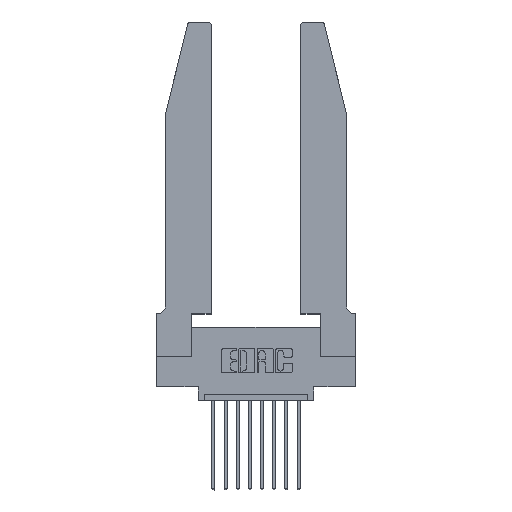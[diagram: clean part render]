
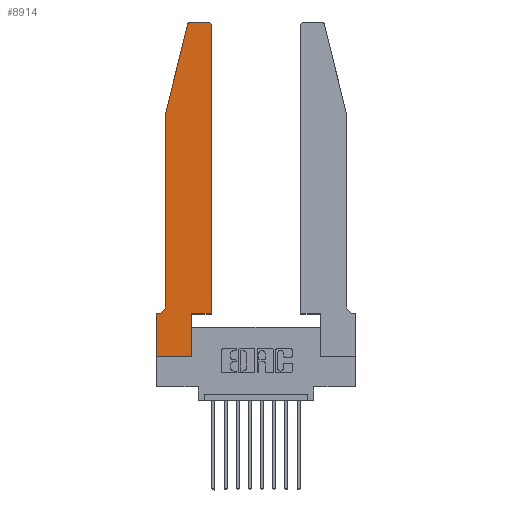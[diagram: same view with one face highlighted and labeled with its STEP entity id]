
A CAD part, top view. The second image highlights one B-rep face of the part: STEP entity #8914.
In plain terms, the highlighted planar face has unit normal (0, 0, 1).
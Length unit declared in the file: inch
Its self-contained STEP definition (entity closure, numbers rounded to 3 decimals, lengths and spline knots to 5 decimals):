
#703 = DIRECTION ( 'NONE',  ( 1., 0., 0. ) ) ;
#865 = VECTOR ( 'NONE', #4171, 39.37008 ) ;
#1129 = CARTESIAN_POINT ( 'NONE',  ( 0.284, 2.72, 0.37 ) ) ;
#1334 = ORIENTED_EDGE ( 'NONE', *, *, #7457, .T. ) ;
#1500 = ORIENTED_EDGE ( 'NONE', *, *, #13188, .T. ) ;
#1532 = CARTESIAN_POINT ( 'NONE',  ( 0.0755, 0.42, 0.37 ) ) ;
#1730 = CIRCLE ( 'NONE', #3489, 0.03 ) ;
#1810 = CARTESIAN_POINT ( 'NONE',  ( 0., 0., 0.37 ) ) ;
#2021 = DIRECTION ( 'NONE',  ( 0., 0., 1. ) ) ;
#2059 = LINE ( 'NONE', #1810, #7297 ) ;
#2123 = ORIENTED_EDGE ( 'NONE', *, *, #7817, .T. ) ;
#2162 = CARTESIAN_POINT ( 'NONE',  ( 0.2865, 0.35, 0.37 ) ) ;
#2186 = DIRECTION ( 'NONE',  ( -1., 0., 0. ) ) ;
#2291 = EDGE_LOOP ( 'NONE', ( #1500, #11821, #11492, #4103, #11208, #12050, #1334, #4428, #11023, #2123, #2442, #6699 ) ) ;
#2324 = CARTESIAN_POINT ( 'NONE',  ( 0.4205, 2.75, 0.37 ) ) ;
#2404 = DIRECTION ( 'NONE',  ( 0., 1., 0. ) ) ;
#2442 = ORIENTED_EDGE ( 'NONE', *, *, #6594, .T. ) ;
#2480 = CARTESIAN_POINT ( 'NONE',  ( 0.0755, 2., 0.37 ) ) ;
#2630 = CARTESIAN_POINT ( 'NONE',  ( 0., 0., 0.37 ) ) ;
#2675 = CARTESIAN_POINT ( 'NONE',  ( 0., 0., 0.37 ) ) ;
#2876 = VECTOR ( 'NONE', #4924, 39.37008 ) ;
#3134 = VECTOR ( 'NONE', #4194, 39.37008 ) ;
#3347 = VERTEX_POINT ( 'NONE', #7876 ) ;
#3489 = AXIS2_PLACEMENT_3D ( 'NONE', #6649, #2021, #703 ) ;
#3671 = FACE_OUTER_BOUND ( 'NONE', #2291, .T. ) ;
#4103 = ORIENTED_EDGE ( 'NONE', *, *, #8977, .T. ) ;
#4171 = DIRECTION ( 'NONE',  ( 0., -1., 0. ) ) ;
#4194 = DIRECTION ( 'NONE',  ( 0., 1., 0. ) ) ;
#4280 = EDGE_CURVE ( 'NONE', #15359, #8386, #5883, .T. ) ;
#4428 = ORIENTED_EDGE ( 'NONE', *, *, #14507, .T. ) ;
#4581 = AXIS2_PLACEMENT_3D ( 'NONE', #5215, #9995, #13709 ) ;
#4614 = VERTEX_POINT ( 'NONE', #8157 ) ;
#4744 = DIRECTION ( 'NONE',  ( -1., 0., 0. ) ) ;
#4924 = DIRECTION ( 'NONE',  ( -0.239, -0.971, 0. ) ) ;
#4974 = CARTESIAN_POINT ( 'NONE',  ( 0.4505, 0.35, 0.37 ) ) ;
#5093 = VECTOR ( 'NONE', #2404, 39.37008 ) ;
#5166 = CARTESIAN_POINT ( 'NONE',  ( 0.0055, 0.35, 0.37 ) ) ;
#5215 = CARTESIAN_POINT ( 'NONE',  ( 0.0055, 0.42, 0.37 ) ) ;
#5605 = CARTESIAN_POINT ( 'NONE',  ( 0., 0.35, 0.37 ) ) ;
#5632 = EDGE_CURVE ( 'NONE', #3347, #9350, #1730, .T. ) ;
#5797 = EDGE_CURVE ( 'NONE', #4614, #12035, #6051, .T. ) ;
#5883 = CIRCLE ( 'NONE', #4581, 0.07 ) ;
#5971 = DIRECTION ( 'NONE',  ( 1., 0., 0. ) ) ;
#5994 = LINE ( 'NONE', #2675, #7677 ) ;
#6051 = LINE ( 'NONE', #7262, #2876 ) ;
#6124 = DIRECTION ( 'NONE',  ( 0., 0., 1. ) ) ;
#6227 = VERTEX_POINT ( 'NONE', #13245 ) ;
#6325 = LINE ( 'NONE', #6650, #3134 ) ;
#6479 = CARTESIAN_POINT ( 'NONE',  ( 0., 0.35, 0.37 ) ) ;
#6594 = EDGE_CURVE ( 'NONE', #14875, #3347, #8634, .T. ) ;
#6649 = CARTESIAN_POINT ( 'NONE',  ( 0.4205, 2.72, 0.37 ) ) ;
#6650 = CARTESIAN_POINT ( 'NONE',  ( 0.2865, 0.35, 0.37 ) ) ;
#6699 = ORIENTED_EDGE ( 'NONE', *, *, #5632, .T. ) ;
#6800 = DIRECTION ( 'NONE',  ( 1., 0., 0. ) ) ;
#6939 = LINE ( 'NONE', #9329, #9908 ) ;
#7262 = CARTESIAN_POINT ( 'NONE',  ( 0.0755, 2., 0.37 ) ) ;
#7297 = VECTOR ( 'NONE', #8869, 39.37008 ) ;
#7308 = VECTOR ( 'NONE', #4744, 39.37008 ) ;
#7457 = EDGE_CURVE ( 'NONE', #13392, #14894, #5994, .T. ) ;
#7660 = VECTOR ( 'NONE', #5971, 39.37008 ) ;
#7677 = VECTOR ( 'NONE', #12021, 39.37008 ) ;
#7817 = EDGE_CURVE ( 'NONE', #14846, #14875, #9886, .T. ) ;
#7876 = CARTESIAN_POINT ( 'NONE',  ( 0.4505, 2.72, 0.37 ) ) ;
#8157 = CARTESIAN_POINT ( 'NONE',  ( 0.25487, 2.72718, 0.37 ) ) ;
#8386 = VERTEX_POINT ( 'NONE', #5166 ) ;
#8634 = LINE ( 'NONE', #4974, #5093 ) ;
#8869 = DIRECTION ( 'NONE',  ( 1., 0., 0. ) ) ;
#8914 = ADVANCED_FACE ( 'NONE', ( #3671 ), #11519, .T. ) ;
#8977 = EDGE_CURVE ( 'NONE', #12035, #15359, #13587, .T. ) ;
#9088 = EDGE_CURVE ( 'NONE', #9193, #14846, #6325, .T. ) ;
#9178 = CARTESIAN_POINT ( 'NONE',  ( 0.0755, 2., 0.37 ) ) ;
#9193 = VERTEX_POINT ( 'NONE', #14758 ) ;
#9329 = CARTESIAN_POINT ( 'NONE',  ( 0.2605, 2.75, 0.37 ) ) ;
#9350 = VERTEX_POINT ( 'NONE', #2324 ) ;
#9886 = LINE ( 'NONE', #13187, #7660 ) ;
#9908 = VECTOR ( 'NONE', #2186, 39.37008 ) ;
#9995 = DIRECTION ( 'NONE',  ( 0., 0., -1. ) ) ;
#10645 = LINE ( 'NONE', #12028, #7308 ) ;
#10739 = DIRECTION ( 'NONE',  ( 1., 0., 0. ) ) ;
#11023 = ORIENTED_EDGE ( 'NONE', *, *, #9088, .T. ) ;
#11053 = AXIS2_PLACEMENT_3D ( 'NONE', #5605, #13994, #6800 ) ;
#11208 = ORIENTED_EDGE ( 'NONE', *, *, #4280, .T. ) ;
#11492 = ORIENTED_EDGE ( 'NONE', *, *, #5797, .T. ) ;
#11519 = PLANE ( 'NONE',  #11053 ) ;
#11821 = ORIENTED_EDGE ( 'NONE', *, *, #12711, .T. ) ;
#12021 = DIRECTION ( 'NONE',  ( 0., -1., 0. ) ) ;
#12028 = CARTESIAN_POINT ( 'NONE',  ( 0.0755, 0.35, 0.37 ) ) ;
#12035 = VERTEX_POINT ( 'NONE', #2480 ) ;
#12050 = ORIENTED_EDGE ( 'NONE', *, *, #13228, .T. ) ;
#12711 = EDGE_CURVE ( 'NONE', #6227, #4614, #14637, .T. ) ;
#12908 = CARTESIAN_POINT ( 'NONE',  ( 0.4505, 0.35, 0.37 ) ) ;
#13187 = CARTESIAN_POINT ( 'NONE',  ( 0.4505, 0.35, 0.37 ) ) ;
#13188 = EDGE_CURVE ( 'NONE', #9350, #6227, #6939, .T. ) ;
#13228 = EDGE_CURVE ( 'NONE', #8386, #13392, #10645, .T. ) ;
#13245 = CARTESIAN_POINT ( 'NONE',  ( 0.284, 2.75, 0.37 ) ) ;
#13392 = VERTEX_POINT ( 'NONE', #6479 ) ;
#13587 = LINE ( 'NONE', #9178, #865 ) ;
#13709 = DIRECTION ( 'NONE',  ( -1., 0., 0. ) ) ;
#13897 = AXIS2_PLACEMENT_3D ( 'NONE', #1129, #6124, #10739 ) ;
#13994 = DIRECTION ( 'NONE',  ( 0., 0., 1. ) ) ;
#14507 = EDGE_CURVE ( 'NONE', #14894, #9193, #2059, .T. ) ;
#14637 = CIRCLE ( 'NONE', #13897, 0.03 ) ;
#14758 = CARTESIAN_POINT ( 'NONE',  ( 0.2865, 0., 0.37 ) ) ;
#14846 = VERTEX_POINT ( 'NONE', #2162 ) ;
#14875 = VERTEX_POINT ( 'NONE', #12908 ) ;
#14894 = VERTEX_POINT ( 'NONE', #2630 ) ;
#15359 = VERTEX_POINT ( 'NONE', #1532 ) ;
